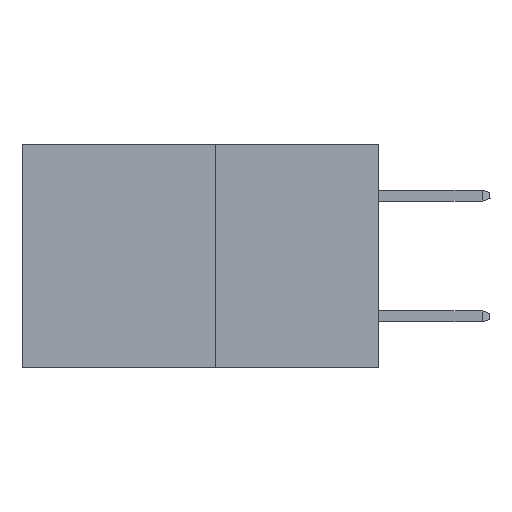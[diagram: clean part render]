
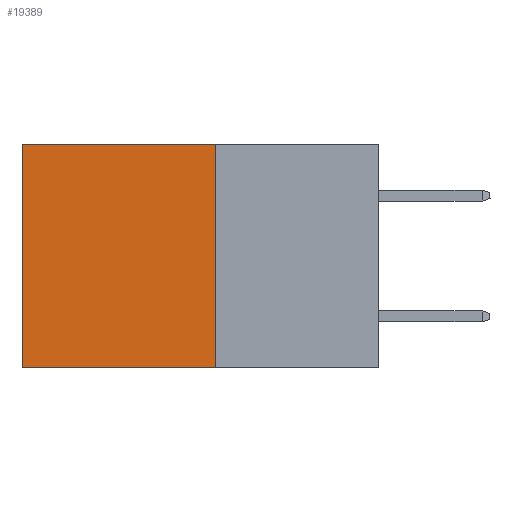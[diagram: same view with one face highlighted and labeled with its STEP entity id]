
A CAD part, left-side view. The second image highlights one B-rep face of the part: STEP entity #19389.
In plain terms, the highlighted planar face has unit normal (-1, 0, 0).
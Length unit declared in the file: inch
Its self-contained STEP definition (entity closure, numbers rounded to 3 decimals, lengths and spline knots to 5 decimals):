
#1774 = LINE ( 'NONE', #10297, #24346 ) ;
#3557 = CARTESIAN_POINT ( 'NONE',  ( 0.277, 0.59, 0. ) ) ;
#4524 = ORIENTED_EDGE ( 'NONE', *, *, #24369, .T. ) ;
#4540 = ORIENTED_EDGE ( 'NONE', *, *, #10452, .F. ) ;
#4677 = DIRECTION ( 'NONE',  ( 0., 1., 0. ) ) ;
#5866 = CARTESIAN_POINT ( 'NONE',  ( 0.277, 0.27, -0.37 ) ) ;
#6036 = AXIS2_PLACEMENT_3D ( 'NONE', #7267, #24767, #11758 ) ;
#6919 = CARTESIAN_POINT ( 'NONE',  ( 0.277, 0.27, -0.37 ) ) ;
#7267 = CARTESIAN_POINT ( 'NONE',  ( 0.277, 0.27, -0.37 ) ) ;
#8131 = DIRECTION ( 'NONE',  ( 0., 0., -1. ) ) ;
#8214 = VERTEX_POINT ( 'NONE', #3557 ) ;
#8242 = EDGE_CURVE ( 'NONE', #20226, #10819, #17482, .T. ) ;
#9177 = ORIENTED_EDGE ( 'NONE', *, *, #11809, .T. ) ;
#9322 = VECTOR ( 'NONE', #4677, 39.37008 ) ;
#9744 = LINE ( 'NONE', #26157, #17068 ) ;
#10175 = VECTOR ( 'NONE', #19082, 39.37008 ) ;
#10297 = CARTESIAN_POINT ( 'NONE',  ( 0.277, 0.59, -0.37 ) ) ;
#10452 = EDGE_CURVE ( 'NONE', #13571, #20226, #9744, .T. ) ;
#10819 = VERTEX_POINT ( 'NONE', #22505 ) ;
#10986 = DIRECTION ( 'NONE',  ( 0., 0., -1. ) ) ;
#11758 = DIRECTION ( 'NONE',  ( 0., 0., -1. ) ) ;
#11809 = EDGE_CURVE ( 'NONE', #8214, #10819, #1774, .T. ) ;
#13571 = VERTEX_POINT ( 'NONE', #21237 ) ;
#17068 = VECTOR ( 'NONE', #10986, 39.37008 ) ;
#17482 = LINE ( 'NONE', #5866, #10175 ) ;
#18402 = FACE_OUTER_BOUND ( 'NONE', #27660, .T. ) ;
#19082 = DIRECTION ( 'NONE',  ( 0., 1., 0. ) ) ;
#19389 = ADVANCED_FACE ( 'NONE', ( #18402 ), #22623, .F. ) ;
#20083 = CARTESIAN_POINT ( 'NONE',  ( 0.277, 0.27, 0. ) ) ;
#20226 = VERTEX_POINT ( 'NONE', #6919 ) ;
#21021 = LINE ( 'NONE', #20083, #9322 ) ;
#21237 = CARTESIAN_POINT ( 'NONE',  ( 0.277, 0.27, 0. ) ) ;
#22505 = CARTESIAN_POINT ( 'NONE',  ( 0.277, 0.59, -0.37 ) ) ;
#22623 = PLANE ( 'NONE',  #6036 ) ;
#23306 = ORIENTED_EDGE ( 'NONE', *, *, #8242, .F. ) ;
#24346 = VECTOR ( 'NONE', #8131, 39.37008 ) ;
#24369 = EDGE_CURVE ( 'NONE', #13571, #8214, #21021, .T. ) ;
#24767 = DIRECTION ( 'NONE',  ( 1., 0., 0. ) ) ;
#26157 = CARTESIAN_POINT ( 'NONE',  ( 0.277, 0.27, -0.37 ) ) ;
#27660 = EDGE_LOOP ( 'NONE', ( #9177, #23306, #4540, #4524 ) ) ;
